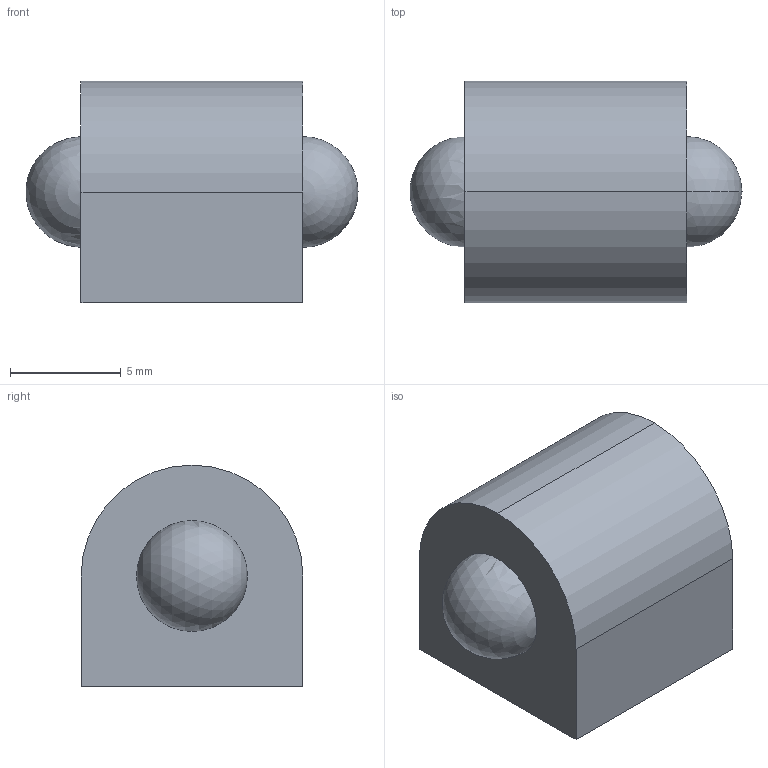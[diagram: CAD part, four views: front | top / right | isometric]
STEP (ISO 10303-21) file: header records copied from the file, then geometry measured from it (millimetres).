
FILE_DESCRIPTION (( 'STEP AP214' ), '1' );
FILE_NAME ('Rubber_Band_Connecter.step', '2013-11-06T14:31:16', ( 'elpi' ), ( '' ), 'SwSTEP 2.0', 'SolidWorks 2013', '' );
FILE_SCHEMA (( 'AUTOMOTIVE_DESIGN' ));
Length unit declared in the file: millimetre
Products named in the file (1): Rubber_Band_Connecter
Bounding box: 14.98 x 10 x 10 mm (x, y, z)
Volume: 958.1 mm3; surface area: 574.9 mm2
Topology: 1 solids, 1 shells, 10 faces, 28 edges, 18 vertices
Faces by surface type: plane 5, sphere 3, cylinder 2
Entity records: 303 total; most frequent: DIRECTION 51, CARTESIAN_POINT 45, ORIENTED_EDGE 40, EDGE_CURVE 20, AXIS2_PLACEMENT_3D 20, VERTEX_POINT 14, EDGE_LOOP 12, VECTOR 11
